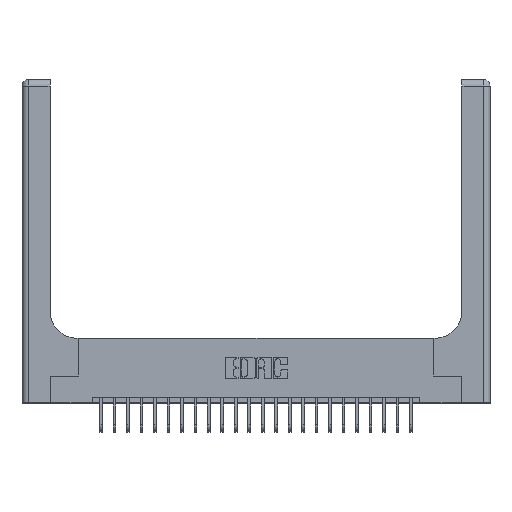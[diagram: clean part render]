
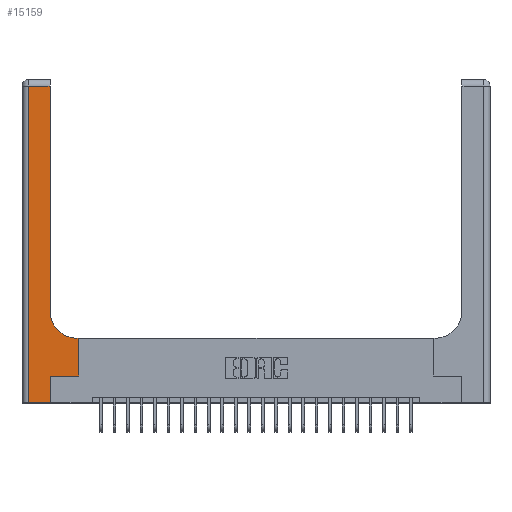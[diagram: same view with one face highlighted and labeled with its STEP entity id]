
A CAD part, top view. The second image highlights one B-rep face of the part: STEP entity #15159.
In plain terms, the highlighted planar face has unit normal (0, 0, 1).
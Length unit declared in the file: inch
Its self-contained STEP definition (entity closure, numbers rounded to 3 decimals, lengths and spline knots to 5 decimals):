
#453 = ORIENTED_EDGE ( 'NONE', *, *, #22528, .T. ) ;
#949 = VERTEX_POINT ( 'NONE', #6863 ) ;
#1651 = ORIENTED_EDGE ( 'NONE', *, *, #5103, .T. ) ;
#1720 = VECTOR ( 'NONE', #22769, 39.37008 ) ;
#2033 = EDGE_CURVE ( 'NONE', #3382, #10133, #11018, .T. ) ;
#2119 = EDGE_CURVE ( 'NONE', #4441, #3382, #11236, .T. ) ;
#2157 = ORIENTED_EDGE ( 'NONE', *, *, #4049, .T. ) ;
#2391 = CARTESIAN_POINT ( 'NONE',  ( 0.528, 0.25, 0.37 ) ) ;
#2487 = EDGE_CURVE ( 'NONE', #18164, #19742, #11671, .T. ) ;
#2696 = CARTESIAN_POINT ( 'NONE',  ( 0., 0., 0.37 ) ) ;
#2969 = VECTOR ( 'NONE', #18434, 39.37008 ) ;
#3382 = VERTEX_POINT ( 'NONE', #9479 ) ;
#3882 = VECTOR ( 'NONE', #14377, 39.37008 ) ;
#4049 = EDGE_CURVE ( 'NONE', #20947, #4441, #18178, .T. ) ;
#4206 = DIRECTION ( 'NONE',  ( -1., 0., 0. ) ) ;
#4441 = VERTEX_POINT ( 'NONE', #6378 ) ;
#5103 = EDGE_CURVE ( 'NONE', #949, #9796, #6185, .T. ) ;
#5782 = CARTESIAN_POINT ( 'NONE',  ( 0.26, 0.85, 0.37 ) ) ;
#6185 = LINE ( 'NONE', #2696, #2969 ) ;
#6378 = CARTESIAN_POINT ( 'NONE',  ( 0.528, 0.25, 0.37 ) ) ;
#6863 = CARTESIAN_POINT ( 'NONE',  ( 0.06, 0., 0.37 ) ) ;
#7505 = CARTESIAN_POINT ( 'NONE',  ( 0.26, 0.6, 0.37 ) ) ;
#7883 = CARTESIAN_POINT ( 'NONE',  ( 0.26, 2.94, 0.37 ) ) ;
#7904 = FACE_OUTER_BOUND ( 'NONE', #22428, .T. ) ;
#8452 = ORIENTED_EDGE ( 'NONE', *, *, #20933, .T. ) ;
#8566 = LINE ( 'NONE', #13915, #1720 ) ;
#9216 = VECTOR ( 'NONE', #4206, 39.37008 ) ;
#9360 = ORIENTED_EDGE ( 'NONE', *, *, #2033, .T. ) ;
#9479 = CARTESIAN_POINT ( 'NONE',  ( 0.528, 0.6, 0.37 ) ) ;
#9796 = VERTEX_POINT ( 'NONE', #10684 ) ;
#9885 = AXIS2_PLACEMENT_3D ( 'NONE', #22119, #20505, #22360 ) ;
#9887 = ORIENTED_EDGE ( 'NONE', *, *, #2119, .T. ) ;
#10073 = VERTEX_POINT ( 'NONE', #5782 ) ;
#10133 = VERTEX_POINT ( 'NONE', #11369 ) ;
#10164 = CARTESIAN_POINT ( 'NONE',  ( 0.06, 3., 0.37 ) ) ;
#10277 = LINE ( 'NONE', #10164, #13924 ) ;
#10684 = CARTESIAN_POINT ( 'NONE',  ( 0.265, 0., 0.37 ) ) ;
#10955 = VECTOR ( 'NONE', #16063, 39.37008 ) ;
#11018 = LINE ( 'NONE', #7505, #21716 ) ;
#11236 = LINE ( 'NONE', #2391, #3882 ) ;
#11369 = CARTESIAN_POINT ( 'NONE',  ( 0.51, 0.6, 0.37 ) ) ;
#11671 = LINE ( 'NONE', #15046, #9216 ) ;
#12438 = EDGE_CURVE ( 'NONE', #19742, #949, #10277, .T. ) ;
#13915 = CARTESIAN_POINT ( 'NONE',  ( 0.265, 0., 0.37 ) ) ;
#13924 = VECTOR ( 'NONE', #15174, 39.37008 ) ;
#14377 = DIRECTION ( 'NONE',  ( 0., 1., 0. ) ) ;
#15046 = CARTESIAN_POINT ( 'NONE',  ( 0., 2.94, 0.37 ) ) ;
#15050 = ORIENTED_EDGE ( 'NONE', *, *, #21083, .T. ) ;
#15135 = ORIENTED_EDGE ( 'NONE', *, *, #2487, .T. ) ;
#15159 = ADVANCED_FACE ( 'NONE', ( #7904 ), #15253, .F. ) ;
#15174 = DIRECTION ( 'NONE',  ( 0., -1., 0. ) ) ;
#15253 = PLANE ( 'NONE',  #9885 ) ;
#15439 = CARTESIAN_POINT ( 'NONE',  ( 0.06, 2.94, 0.37 ) ) ;
#16063 = DIRECTION ( 'NONE',  ( 1., 0., 0. ) ) ;
#16293 = AXIS2_PLACEMENT_3D ( 'NONE', #20674, #22054, #20440 ) ;
#17774 = CIRCLE ( 'NONE', #16293, 0.25 ) ;
#18002 = LINE ( 'NONE', #21719, #19968 ) ;
#18164 = VERTEX_POINT ( 'NONE', #7883 ) ;
#18178 = LINE ( 'NONE', #19578, #10955 ) ;
#18434 = DIRECTION ( 'NONE',  ( 1., 0., 0. ) ) ;
#18466 = DIRECTION ( 'NONE',  ( -1., 0., 0. ) ) ;
#19578 = CARTESIAN_POINT ( 'NONE',  ( 0.265, 0.25, 0.37 ) ) ;
#19638 = DIRECTION ( 'NONE',  ( 0., 1., 0. ) ) ;
#19742 = VERTEX_POINT ( 'NONE', #15439 ) ;
#19968 = VECTOR ( 'NONE', #19638, 39.37008 ) ;
#20398 = ORIENTED_EDGE ( 'NONE', *, *, #12438, .T. ) ;
#20440 = DIRECTION ( 'NONE',  ( 1., 0., 0. ) ) ;
#20505 = DIRECTION ( 'NONE',  ( 0., 0., -1. ) ) ;
#20674 = CARTESIAN_POINT ( 'NONE',  ( 0.51, 0.85, 0.37 ) ) ;
#20933 = EDGE_CURVE ( 'NONE', #9796, #20947, #8566, .T. ) ;
#20947 = VERTEX_POINT ( 'NONE', #21151 ) ;
#21083 = EDGE_CURVE ( 'NONE', #10073, #18164, #18002, .T. ) ;
#21151 = CARTESIAN_POINT ( 'NONE',  ( 0.265, 0.25, 0.37 ) ) ;
#21716 = VECTOR ( 'NONE', #18466, 39.37008 ) ;
#21719 = CARTESIAN_POINT ( 'NONE',  ( 0.26, 3., 0.37 ) ) ;
#22054 = DIRECTION ( 'NONE',  ( 0., 0., -1. ) ) ;
#22119 = CARTESIAN_POINT ( 'NONE',  ( 0., 3., 0.37 ) ) ;
#22360 = DIRECTION ( 'NONE',  ( -1., 0., 0. ) ) ;
#22428 = EDGE_LOOP ( 'NONE', ( #15050, #15135, #20398, #1651, #8452, #2157, #9887, #9360, #453 ) ) ;
#22528 = EDGE_CURVE ( 'NONE', #10133, #10073, #17774, .T. ) ;
#22769 = DIRECTION ( 'NONE',  ( 0., 1., 0. ) ) ;
